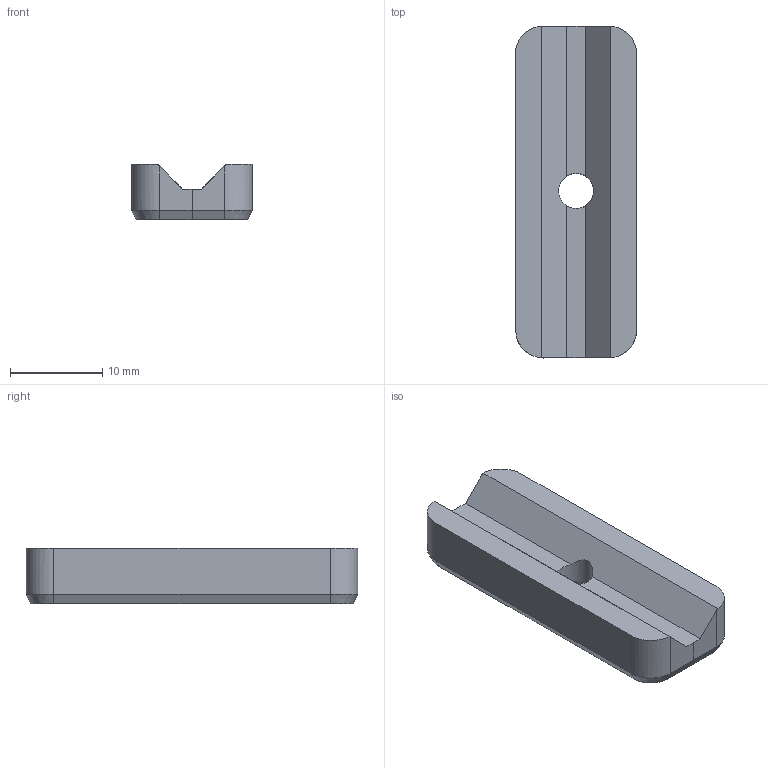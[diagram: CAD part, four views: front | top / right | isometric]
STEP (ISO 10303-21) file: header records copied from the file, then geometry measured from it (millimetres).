
FILE_DESCRIPTION(/* description */ (''),/* implementation_level */ '2;1');
FILE_NAME(/* name */ 'LPL QD Claw.step',/* time_stamp */ '2022-10-11T20:35:37-05:00',/* author */ (''),/* organization */ (''),/* preprocessor_version */ 'ST-DEVELOPER v19',/* originating_system */ 'Autodesk Translation Framework v11.7.0.108',/* authorisation */ '');
FILE_SCHEMA (('AUTOMOTIVE_DESIGN { 1 0 10303 214 3 1 1 }'));
Length unit declared in the file: millimetre
Products named in the file (1): LPL Optic Mount
Bounding box: 13.11 x 36 x 6 mm (x, y, z)
Volume: 2258.6 mm3; surface area: 1520.4 mm2
Topology: 1 solids, 1 shells, 29 faces, 73 edges, 45 vertices
Faces by surface type: plane 19, cylinder 5, cone 5
Full cylindrical faces by diameter (mm): 3.8 x1
Entity records: 899 total; most frequent: DIRECTION 156, CARTESIAN_POINT 148, ORIENTED_EDGE 146, EDGE_CURVE 73, AXIS2_PLACEMENT_3D 53, LINE 50, VECTOR 50, VERTEX_POINT 45
